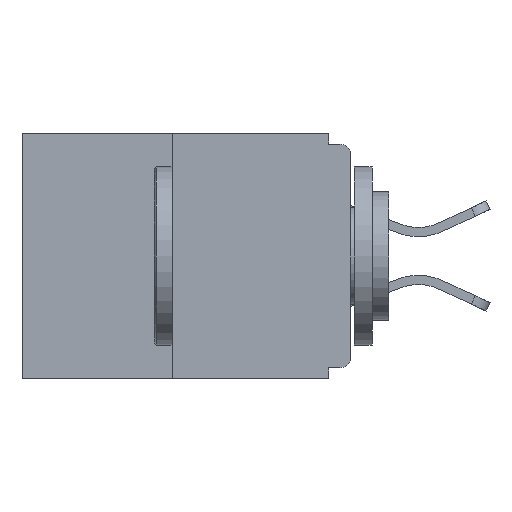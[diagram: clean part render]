
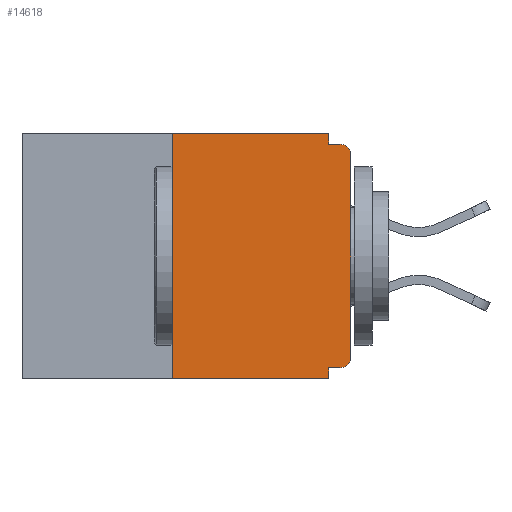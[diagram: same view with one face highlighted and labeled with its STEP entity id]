
A CAD part, left-side view. The second image highlights one B-rep face of the part: STEP entity #14618.
In plain terms, the highlighted planar face has unit normal (-1, 0, 0).
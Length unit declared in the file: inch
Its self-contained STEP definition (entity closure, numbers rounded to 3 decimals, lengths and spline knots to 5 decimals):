
#530 = VECTOR ( 'NONE', #17198, 39.37008 ) ;
#900 = CARTESIAN_POINT ( 'NONE',  ( 0., 0.015, -0.015 ) ) ;
#1069 = VECTOR ( 'NONE', #20676, 39.37008 ) ;
#1164 = LINE ( 'NONE', #12671, #8521 ) ;
#1255 = AXIS2_PLACEMENT_3D ( 'NONE', #5902, #1709, #11834 ) ;
#1489 = ORIENTED_EDGE ( 'NONE', *, *, #17605, .F. ) ;
#1709 = DIRECTION ( 'NONE',  ( -1., 0., 0. ) ) ;
#1832 = DIRECTION ( 'NONE',  ( 0., 0., -1. ) ) ;
#1907 = DIRECTION ( 'NONE',  ( 0., 0., -1. ) ) ;
#1924 = VERTEX_POINT ( 'NONE', #6498 ) ;
#2863 = CARTESIAN_POINT ( 'NONE',  ( 0., 0., -0.328 ) ) ;
#3309 = VERTEX_POINT ( 'NONE', #900 ) ;
#3457 = CARTESIAN_POINT ( 'NONE',  ( 0., 0.015, -0.328 ) ) ;
#3535 = DIRECTION ( 'NONE',  ( 0., 0., 1. ) ) ;
#3592 = CARTESIAN_POINT ( 'NONE',  ( 0., 0.031, -0.343 ) ) ;
#3712 = CARTESIAN_POINT ( 'NONE',  ( 0., 0., 0. ) ) ;
#4086 = DIRECTION ( 'NONE',  ( -1., 0., 0. ) ) ;
#4762 = VERTEX_POINT ( 'NONE', #3457 ) ;
#5655 = CARTESIAN_POINT ( 'NONE',  ( 0., 0.46, 0. ) ) ;
#5854 = CARTESIAN_POINT ( 'NONE',  ( 0., 0.015, -0.313 ) ) ;
#5902 = CARTESIAN_POINT ( 'NONE',  ( 0., 0.015, -0.03 ) ) ;
#5974 = ORIENTED_EDGE ( 'NONE', *, *, #8384, .F. ) ;
#6092 = LINE ( 'NONE', #19790, #19575 ) ;
#6494 = EDGE_CURVE ( 'NONE', #13371, #23615, #13469, .T. ) ;
#6498 = CARTESIAN_POINT ( 'NONE',  ( 0., 0., -0.313 ) ) ;
#6949 = CARTESIAN_POINT ( 'NONE',  ( 0., 0., -0.03 ) ) ;
#7391 = VERTEX_POINT ( 'NONE', #20211 ) ;
#7770 = LINE ( 'NONE', #26256, #1069 ) ;
#7910 = PLANE ( 'NONE',  #21835 ) ;
#8384 = EDGE_CURVE ( 'NONE', #4762, #13371, #20776, .T. ) ;
#8521 = VECTOR ( 'NONE', #21035, 39.37008 ) ;
#8740 = EDGE_CURVE ( 'NONE', #9252, #3309, #1164, .T. ) ;
#9099 = CARTESIAN_POINT ( 'NONE',  ( 0., 0.25, 0. ) ) ;
#9252 = VERTEX_POINT ( 'NONE', #21225 ) ;
#9361 = LINE ( 'NONE', #3712, #16416 ) ;
#10332 = DIRECTION ( 'NONE',  ( 0., 0., -1. ) ) ;
#11674 = CARTESIAN_POINT ( 'NONE',  ( 0., 0.031, -0.328 ) ) ;
#11834 = DIRECTION ( 'NONE',  ( 0., 0., -1. ) ) ;
#12062 = VERTEX_POINT ( 'NONE', #25221 ) ;
#12671 = CARTESIAN_POINT ( 'NONE',  ( 0., 0., -0.015 ) ) ;
#12742 = EDGE_CURVE ( 'NONE', #12062, #23615, #6092, .T. ) ;
#12814 = VECTOR ( 'NONE', #1907, 39.37008 ) ;
#12940 = VECTOR ( 'NONE', #19824, 39.37008 ) ;
#13141 = VECTOR ( 'NONE', #14936, 39.37008 ) ;
#13163 = ORIENTED_EDGE ( 'NONE', *, *, #6494, .F. ) ;
#13371 = VERTEX_POINT ( 'NONE', #11674 ) ;
#13469 = LINE ( 'NONE', #16059, #12814 ) ;
#14104 = CARTESIAN_POINT ( 'NONE',  ( 0., 0.46, 0. ) ) ;
#14232 = LINE ( 'NONE', #5655, #12940 ) ;
#14566 = EDGE_CURVE ( 'NONE', #4762, #1924, #17247, .T. ) ;
#14618 = ADVANCED_FACE ( 'NONE', ( #25626 ), #7910, .F. ) ;
#14936 = DIRECTION ( 'NONE',  ( 0., 0., 1. ) ) ;
#15443 = AXIS2_PLACEMENT_3D ( 'NONE', #5854, #4086, #10332 ) ;
#15649 = DIRECTION ( 'NONE',  ( 0., -1., 0. ) ) ;
#15943 = ORIENTED_EDGE ( 'NONE', *, *, #19134, .F. ) ;
#16059 = CARTESIAN_POINT ( 'NONE',  ( 0., 0.031, -0.343 ) ) ;
#16416 = VECTOR ( 'NONE', #3535, 39.37008 ) ;
#17198 = DIRECTION ( 'NONE',  ( 0., 1., 0. ) ) ;
#17247 = CIRCLE ( 'NONE', #15443, 0.015 ) ;
#17266 = EDGE_LOOP ( 'NONE', ( #26042, #15943, #21390, #13163, #5974, #19208, #21292, #24938, #20332, #1489 ) ) ;
#17605 = EDGE_CURVE ( 'NONE', #24091, #9252, #7770, .T. ) ;
#17958 = LINE ( 'NONE', #9099, #13141 ) ;
#17959 = EDGE_CURVE ( 'NONE', #1924, #25861, #9361, .T. ) ;
#18149 = DIRECTION ( 'NONE',  ( 1., 0., 0. ) ) ;
#19134 = EDGE_CURVE ( 'NONE', #12062, #7391, #17958, .T. ) ;
#19208 = ORIENTED_EDGE ( 'NONE', *, *, #14566, .T. ) ;
#19575 = VECTOR ( 'NONE', #15649, 39.37008 ) ;
#19790 = CARTESIAN_POINT ( 'NONE',  ( 0., 0.46, -0.343 ) ) ;
#19824 = DIRECTION ( 'NONE',  ( 0., -1., 0. ) ) ;
#20211 = CARTESIAN_POINT ( 'NONE',  ( 0., 0.25, 0. ) ) ;
#20332 = ORIENTED_EDGE ( 'NONE', *, *, #8740, .F. ) ;
#20676 = DIRECTION ( 'NONE',  ( 0., 0., -1. ) ) ;
#20776 = LINE ( 'NONE', #2863, #530 ) ;
#21035 = DIRECTION ( 'NONE',  ( 0., -1., 0. ) ) ;
#21225 = CARTESIAN_POINT ( 'NONE',  ( 0., 0.031, -0.015 ) ) ;
#21292 = ORIENTED_EDGE ( 'NONE', *, *, #17959, .T. ) ;
#21390 = ORIENTED_EDGE ( 'NONE', *, *, #12742, .T. ) ;
#21731 = CIRCLE ( 'NONE', #1255, 0.015 ) ;
#21835 = AXIS2_PLACEMENT_3D ( 'NONE', #14104, #18149, #1832 ) ;
#22072 = EDGE_CURVE ( 'NONE', #7391, #24091, #14232, .T. ) ;
#22977 = EDGE_CURVE ( 'NONE', #25861, #3309, #21731, .T. ) ;
#23615 = VERTEX_POINT ( 'NONE', #3592 ) ;
#24091 = VERTEX_POINT ( 'NONE', #25994 ) ;
#24938 = ORIENTED_EDGE ( 'NONE', *, *, #22977, .T. ) ;
#25221 = CARTESIAN_POINT ( 'NONE',  ( 0., 0.25, -0.343 ) ) ;
#25626 = FACE_OUTER_BOUND ( 'NONE', #17266, .T. ) ;
#25861 = VERTEX_POINT ( 'NONE', #6949 ) ;
#25994 = CARTESIAN_POINT ( 'NONE',  ( 0., 0.031, 0. ) ) ;
#26042 = ORIENTED_EDGE ( 'NONE', *, *, #22072, .F. ) ;
#26256 = CARTESIAN_POINT ( 'NONE',  ( 0., 0.031, 0. ) ) ;
